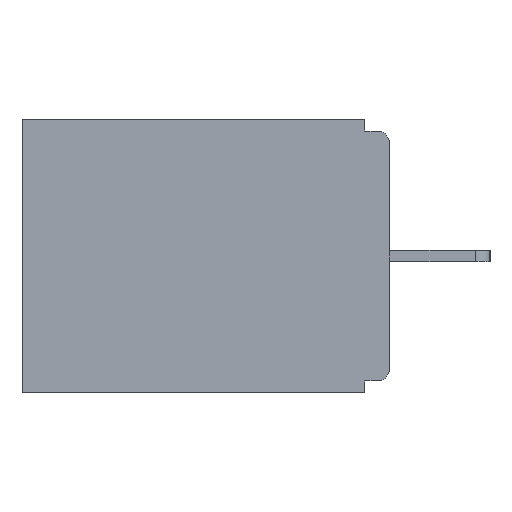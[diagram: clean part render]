
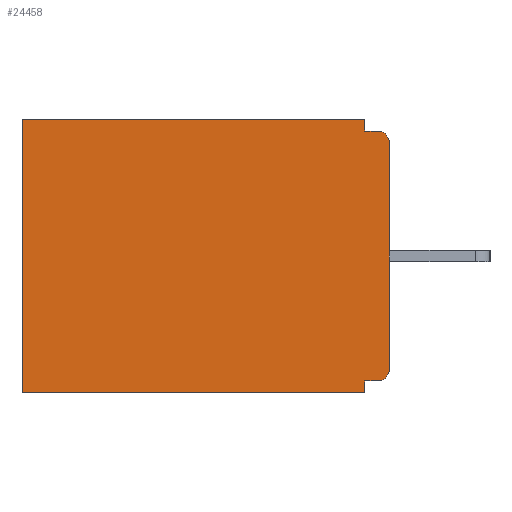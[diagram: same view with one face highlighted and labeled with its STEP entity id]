
A CAD part, left-side view. The second image highlights one B-rep face of the part: STEP entity #24458.
In plain terms, the highlighted planar face has unit normal (-1, 0, 0).
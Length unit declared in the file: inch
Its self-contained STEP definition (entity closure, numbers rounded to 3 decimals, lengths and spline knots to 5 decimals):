
#512 = DIRECTION ( 'NONE',  ( 1., 0., 0. ) ) ;
#537 = CARTESIAN_POINT ( 'NONE',  ( 0.298, 0., 0. ) ) ;
#1017 = VERTEX_POINT ( 'NONE', #9494 ) ;
#1155 = CARTESIAN_POINT ( 'NONE',  ( 0.298, 0., -0.343 ) ) ;
#1249 = DIRECTION ( 'NONE',  ( 0., 1., 0. ) ) ;
#1639 = AXIS2_PLACEMENT_3D ( 'NONE', #21489, #9610, #23410 ) ;
#1699 = VERTEX_POINT ( 'NONE', #4740 ) ;
#1948 = CARTESIAN_POINT ( 'NONE',  ( 0.298, 0.015, -0.015 ) ) ;
#3254 = VERTEX_POINT ( 'NONE', #12182 ) ;
#3330 = ORIENTED_EDGE ( 'NONE', *, *, #19018, .T. ) ;
#3527 = VERTEX_POINT ( 'NONE', #25918 ) ;
#4140 = DIRECTION ( 'NONE',  ( 0., 1., 0. ) ) ;
#4560 = EDGE_CURVE ( 'NONE', #1017, #15964, #6212, .T. ) ;
#4740 = CARTESIAN_POINT ( 'NONE',  ( 0.298, 0., -0.313 ) ) ;
#4971 = CARTESIAN_POINT ( 'NONE',  ( 0.298, 0.031, 0. ) ) ;
#5561 = LINE ( 'NONE', #7924, #20304 ) ;
#5903 = CARTESIAN_POINT ( 'NONE',  ( 0.298, 0.031, -0.343 ) ) ;
#5949 = EDGE_CURVE ( 'NONE', #12840, #1699, #12547, .T. ) ;
#6212 = LINE ( 'NONE', #1155, #16294 ) ;
#6247 = CARTESIAN_POINT ( 'NONE',  ( 0.298, 0.031, -0.343 ) ) ;
#6764 = ORIENTED_EDGE ( 'NONE', *, *, #23755, .F. ) ;
#6794 = ORIENTED_EDGE ( 'NONE', *, *, #5949, .F. ) ;
#6827 = CIRCLE ( 'NONE', #10959, 0.015 ) ;
#7164 = VECTOR ( 'NONE', #20761, 39.37008 ) ;
#7854 = EDGE_CURVE ( 'NONE', #3254, #16718, #5561, .T. ) ;
#7924 = CARTESIAN_POINT ( 'NONE',  ( 0.298, 0., -0.015 ) ) ;
#8278 = DIRECTION ( 'NONE',  ( 0., 1., 0. ) ) ;
#8603 = VECTOR ( 'NONE', #16444, 39.37008 ) ;
#9371 = DIRECTION ( 'NONE',  ( -1., 0., 0. ) ) ;
#9494 = CARTESIAN_POINT ( 'NONE',  ( 0.298, 0.031, -0.343 ) ) ;
#9610 = DIRECTION ( 'NONE',  ( -1., 0., 0. ) ) ;
#9860 = LINE ( 'NONE', #6247, #8603 ) ;
#10959 = AXIS2_PLACEMENT_3D ( 'NONE', #21252, #9371, #23175 ) ;
#11178 = CARTESIAN_POINT ( 'NONE',  ( 0.298, 0.46, 0. ) ) ;
#11428 = EDGE_CURVE ( 'NONE', #18796, #15964, #23112, .T. ) ;
#12182 = CARTESIAN_POINT ( 'NONE',  ( 0.298, 0.031, -0.015 ) ) ;
#12456 = CARTESIAN_POINT ( 'NONE',  ( 0.298, 0.015, -0.328 ) ) ;
#12539 = CARTESIAN_POINT ( 'NONE',  ( 0.298, 0.46, -0.343 ) ) ;
#12547 = LINE ( 'NONE', #537, #7164 ) ;
#12602 = DIRECTION ( 'NONE',  ( 0., -1., 0. ) ) ;
#12840 = VERTEX_POINT ( 'NONE', #25928 ) ;
#12873 = CARTESIAN_POINT ( 'NONE',  ( 0.298, 0., 0. ) ) ;
#13792 = VECTOR ( 'NONE', #19903, 39.37008 ) ;
#14117 = VERTEX_POINT ( 'NONE', #12456 ) ;
#14864 = DIRECTION ( 'NONE',  ( 0., 0., -1. ) ) ;
#14996 = LINE ( 'NONE', #20192, #25338 ) ;
#15752 = DIRECTION ( 'NONE',  ( 0., 0., -1. ) ) ;
#15964 = VERTEX_POINT ( 'NONE', #12539 ) ;
#16143 = EDGE_CURVE ( 'NONE', #16861, #18796, #14996, .T. ) ;
#16294 = VECTOR ( 'NONE', #1249, 39.37008 ) ;
#16304 = CARTESIAN_POINT ( 'NONE',  ( 0.298, 0., -0.328 ) ) ;
#16444 = DIRECTION ( 'NONE',  ( 0., 0., -1. ) ) ;
#16718 = VERTEX_POINT ( 'NONE', #1948 ) ;
#16861 = VERTEX_POINT ( 'NONE', #4971 ) ;
#16936 = AXIS2_PLACEMENT_3D ( 'NONE', #12873, #512, #14864 ) ;
#17124 = ORIENTED_EDGE ( 'NONE', *, *, #4560, .F. ) ;
#17458 = ORIENTED_EDGE ( 'NONE', *, *, #21530, .F. ) ;
#17706 = ORIENTED_EDGE ( 'NONE', *, *, #7854, .F. ) ;
#17903 = VECTOR ( 'NONE', #15752, 39.37008 ) ;
#18529 = EDGE_CURVE ( 'NONE', #14117, #3527, #24598, .T. ) ;
#18796 = VERTEX_POINT ( 'NONE', #11178 ) ;
#18998 = LINE ( 'NONE', #5903, #13792 ) ;
#19018 = EDGE_CURVE ( 'NONE', #12840, #16718, #23106, .T. ) ;
#19903 = DIRECTION ( 'NONE',  ( 0., 0., -1. ) ) ;
#20061 = VECTOR ( 'NONE', #4140, 39.37008 ) ;
#20192 = CARTESIAN_POINT ( 'NONE',  ( 0.298, 0., 0. ) ) ;
#20304 = VECTOR ( 'NONE', #12602, 39.37008 ) ;
#20761 = DIRECTION ( 'NONE',  ( 0., 0., -1. ) ) ;
#21252 = CARTESIAN_POINT ( 'NONE',  ( 0.298, 0.015, -0.313 ) ) ;
#21292 = ORIENTED_EDGE ( 'NONE', *, *, #18529, .F. ) ;
#21489 = CARTESIAN_POINT ( 'NONE',  ( 0.298, 0.015, -0.03 ) ) ;
#21530 = EDGE_CURVE ( 'NONE', #16861, #3254, #18998, .T. ) ;
#21643 = CARTESIAN_POINT ( 'NONE',  ( 0.298, 0.46, 0. ) ) ;
#21755 = ORIENTED_EDGE ( 'NONE', *, *, #16143, .T. ) ;
#21776 = EDGE_LOOP ( 'NONE', ( #3330, #17706, #17458, #21755, #22997, #17124, #6764, #21292, #25724, #6794 ) ) ;
#22456 = FACE_OUTER_BOUND ( 'NONE', #21776, .T. ) ;
#22572 = PLANE ( 'NONE',  #16936 ) ;
#22997 = ORIENTED_EDGE ( 'NONE', *, *, #11428, .T. ) ;
#23106 = CIRCLE ( 'NONE', #1639, 0.015 ) ;
#23112 = LINE ( 'NONE', #21643, #17903 ) ;
#23175 = DIRECTION ( 'NONE',  ( 0., 0., -1. ) ) ;
#23410 = DIRECTION ( 'NONE',  ( 0., 0., -1. ) ) ;
#23755 = EDGE_CURVE ( 'NONE', #3527, #1017, #9860, .T. ) ;
#24458 = ADVANCED_FACE ( 'NONE', ( #22456 ), #22572, .F. ) ;
#24598 = LINE ( 'NONE', #16304, #20061 ) ;
#25338 = VECTOR ( 'NONE', #8278, 39.37008 ) ;
#25526 = EDGE_CURVE ( 'NONE', #14117, #1699, #6827, .T. ) ;
#25724 = ORIENTED_EDGE ( 'NONE', *, *, #25526, .T. ) ;
#25918 = CARTESIAN_POINT ( 'NONE',  ( 0.298, 0.031, -0.328 ) ) ;
#25928 = CARTESIAN_POINT ( 'NONE',  ( 0.298, 0., -0.03 ) ) ;
